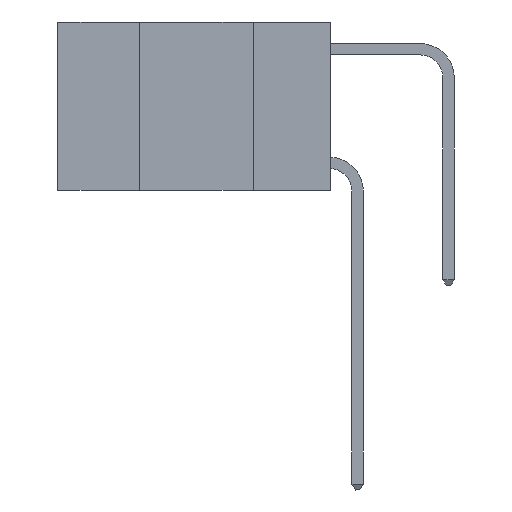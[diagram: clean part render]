
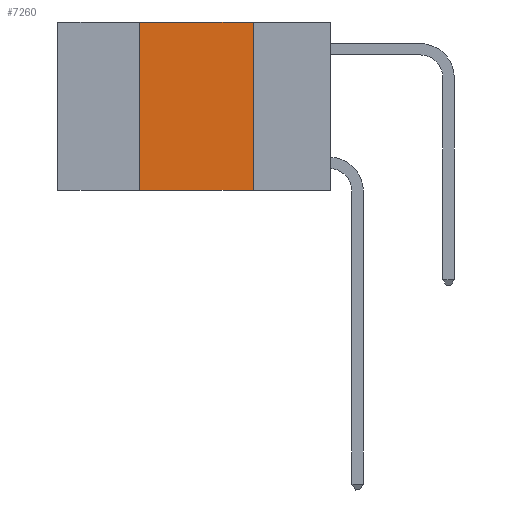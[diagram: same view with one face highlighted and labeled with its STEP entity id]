
A CAD part, left-side view. The second image highlights one B-rep face of the part: STEP entity #7260.
In plain terms, the highlighted planar face has unit normal (-1, 0, 0).
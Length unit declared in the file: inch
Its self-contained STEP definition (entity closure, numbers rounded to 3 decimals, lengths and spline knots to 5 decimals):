
#557 = CARTESIAN_POINT ( 'NONE',  ( 0., 0.17, 0. ) ) ;
#1355 = ORIENTED_EDGE ( 'NONE', *, *, #3850, .T. ) ;
#1589 = EDGE_CURVE ( 'NONE', #9003, #8927, #10880, .T. ) ;
#1773 = PLANE ( 'NONE',  #7196 ) ;
#1853 = LINE ( 'NONE', #1907, #7316 ) ;
#1907 = CARTESIAN_POINT ( 'NONE',  ( 0., 0.42, 0. ) ) ;
#2037 = FACE_OUTER_BOUND ( 'NONE', #5589, .T. ) ;
#2124 = LINE ( 'NONE', #9326, #6444 ) ;
#2453 = ORIENTED_EDGE ( 'NONE', *, *, #3339, .F. ) ;
#2847 = DIRECTION ( 'NONE',  ( 0., 0., 1. ) ) ;
#2916 = CARTESIAN_POINT ( 'NONE',  ( 0., 0.42, -0.37 ) ) ;
#3339 = EDGE_CURVE ( 'NONE', #9802, #9003, #2124, .T. ) ;
#3850 = EDGE_CURVE ( 'NONE', #4101, #8927, #6570, .T. ) ;
#3862 = VECTOR ( 'NONE', #5044, 39.37008 ) ;
#4101 = VERTEX_POINT ( 'NONE', #2916 ) ;
#4916 = ORIENTED_EDGE ( 'NONE', *, *, #1589, .F. ) ;
#4966 = CARTESIAN_POINT ( 'NONE',  ( 0., 0.6, -0.37 ) ) ;
#5044 = DIRECTION ( 'NONE',  ( 0., -1., 0. ) ) ;
#5589 = EDGE_LOOP ( 'NONE', ( #4916, #2453, #11366, #1355 ) ) ;
#6428 = DIRECTION ( 'NONE',  ( 0., 0., -1. ) ) ;
#6444 = VECTOR ( 'NONE', #9263, 39.37008 ) ;
#6570 = LINE ( 'NONE', #4966, #3862 ) ;
#7196 = AXIS2_PLACEMENT_3D ( 'NONE', #7284, #11361, #6428 ) ;
#7260 = ADVANCED_FACE ( 'NONE', ( #2037 ), #1773, .F. ) ;
#7284 = CARTESIAN_POINT ( 'NONE',  ( 0., 0.6, 0. ) ) ;
#7316 = VECTOR ( 'NONE', #2847, 39.37008 ) ;
#7745 = CARTESIAN_POINT ( 'NONE',  ( 0., 0.42, 0. ) ) ;
#8330 = EDGE_CURVE ( 'NONE', #4101, #9802, #1853, .T. ) ;
#8927 = VERTEX_POINT ( 'NONE', #9583 ) ;
#9003 = VERTEX_POINT ( 'NONE', #557 ) ;
#9263 = DIRECTION ( 'NONE',  ( 0., -1., 0. ) ) ;
#9326 = CARTESIAN_POINT ( 'NONE',  ( 0., 0.6, 0. ) ) ;
#9583 = CARTESIAN_POINT ( 'NONE',  ( 0., 0.17, -0.37 ) ) ;
#9802 = VERTEX_POINT ( 'NONE', #7745 ) ;
#9966 = DIRECTION ( 'NONE',  ( 0., 0., -1. ) ) ;
#10066 = CARTESIAN_POINT ( 'NONE',  ( 0., 0.17, 0. ) ) ;
#10650 = VECTOR ( 'NONE', #9966, 39.37008 ) ;
#10880 = LINE ( 'NONE', #10066, #10650 ) ;
#11361 = DIRECTION ( 'NONE',  ( 1., 0., 0. ) ) ;
#11366 = ORIENTED_EDGE ( 'NONE', *, *, #8330, .F. ) ;
